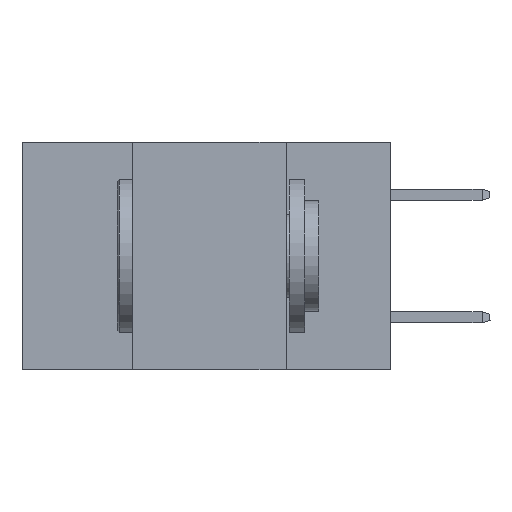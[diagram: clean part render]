
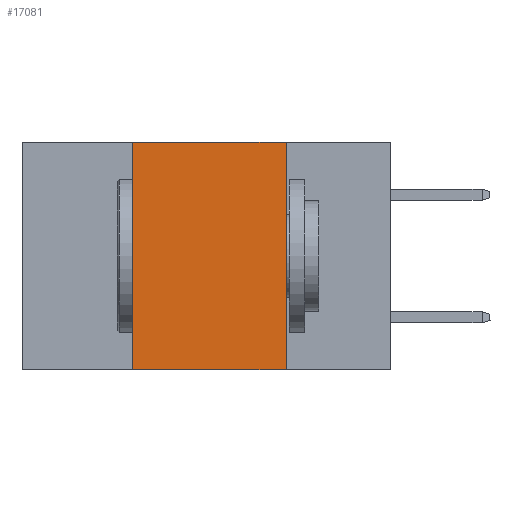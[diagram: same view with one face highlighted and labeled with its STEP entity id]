
A CAD part, left-side view. The second image highlights one B-rep face of the part: STEP entity #17081.
In plain terms, the highlighted planar face has unit normal (-1, 0, 0).
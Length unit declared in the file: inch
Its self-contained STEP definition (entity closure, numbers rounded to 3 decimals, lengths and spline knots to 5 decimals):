
#4513 = ORIENTED_EDGE ( 'NONE', *, *, #28564, .F. ) ;
#4853 = VERTEX_POINT ( 'NONE', #6104 ) ;
#6104 = CARTESIAN_POINT ( 'NONE',  ( 0., 0.17, -0.37 ) ) ;
#7104 = CARTESIAN_POINT ( 'NONE',  ( 0., 0.6, -0.37 ) ) ;
#8259 = ORIENTED_EDGE ( 'NONE', *, *, #15564, .T. ) ;
#8605 = DIRECTION ( 'NONE',  ( 0., 0., -1. ) ) ;
#9020 = VECTOR ( 'NONE', #17049, 39.37008 ) ;
#10167 = CARTESIAN_POINT ( 'NONE',  ( 0., 0.42, -0.37 ) ) ;
#10524 = VERTEX_POINT ( 'NONE', #10167 ) ;
#12477 = ORIENTED_EDGE ( 'NONE', *, *, #30977, .F. ) ;
#12769 = VERTEX_POINT ( 'NONE', #14590 ) ;
#14361 = VECTOR ( 'NONE', #22544, 39.37008 ) ;
#14590 = CARTESIAN_POINT ( 'NONE',  ( 0., 0.17, 0. ) ) ;
#15050 = CARTESIAN_POINT ( 'NONE',  ( 0., 0.6, 0. ) ) ;
#15564 = EDGE_CURVE ( 'NONE', #10524, #4853, #18924, .T. ) ;
#17049 = DIRECTION ( 'NONE',  ( 0., -1., 0. ) ) ;
#17081 = ADVANCED_FACE ( 'NONE', ( #19305 ), #37676, .F. ) ;
#17961 = CARTESIAN_POINT ( 'NONE',  ( 0., 0.42, 0. ) ) ;
#18924 = LINE ( 'NONE', #7104, #9020 ) ;
#19284 = CARTESIAN_POINT ( 'NONE',  ( 0., 0.42, 0. ) ) ;
#19305 = FACE_OUTER_BOUND ( 'NONE', #29488, .T. ) ;
#21806 = CARTESIAN_POINT ( 'NONE',  ( 0., 0.6, 0. ) ) ;
#21901 = VECTOR ( 'NONE', #34444, 39.37008 ) ;
#22544 = DIRECTION ( 'NONE',  ( 0., 0., 1. ) ) ;
#26586 = CARTESIAN_POINT ( 'NONE',  ( 0., 0.17, 0. ) ) ;
#28234 = DIRECTION ( 'NONE',  ( 1., 0., 0. ) ) ;
#28564 = EDGE_CURVE ( 'NONE', #10524, #39439, #39968, .T. ) ;
#29488 = EDGE_LOOP ( 'NONE', ( #36185, #12477, #4513, #8259 ) ) ;
#29797 = DIRECTION ( 'NONE',  ( 0., 0., -1. ) ) ;
#30389 = LINE ( 'NONE', #15050, #21901 ) ;
#30977 = EDGE_CURVE ( 'NONE', #39439, #12769, #30389, .T. ) ;
#32253 = AXIS2_PLACEMENT_3D ( 'NONE', #21806, #28234, #8605 ) ;
#34444 = DIRECTION ( 'NONE',  ( 0., -1., 0. ) ) ;
#36007 = VECTOR ( 'NONE', #29797, 39.37008 ) ;
#36185 = ORIENTED_EDGE ( 'NONE', *, *, #39195, .F. ) ;
#37018 = LINE ( 'NONE', #26586, #36007 ) ;
#37676 = PLANE ( 'NONE',  #32253 ) ;
#39195 = EDGE_CURVE ( 'NONE', #12769, #4853, #37018, .T. ) ;
#39439 = VERTEX_POINT ( 'NONE', #17961 ) ;
#39968 = LINE ( 'NONE', #19284, #14361 ) ;
